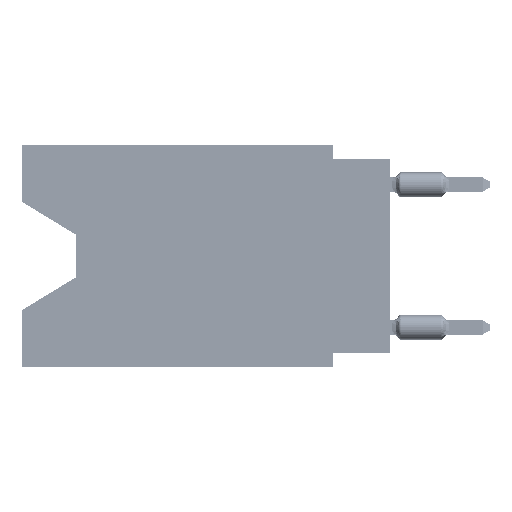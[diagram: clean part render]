
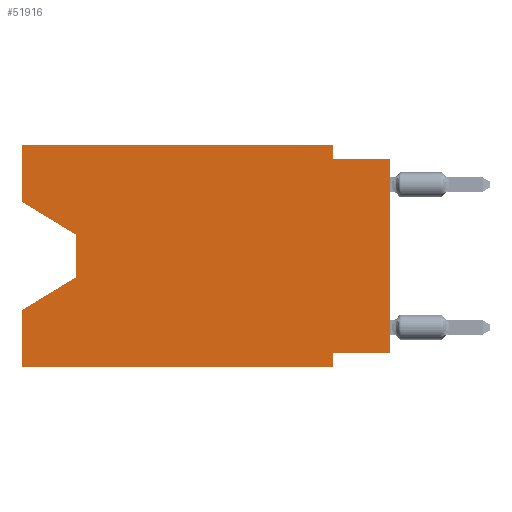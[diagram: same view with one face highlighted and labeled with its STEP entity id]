
A CAD part, left-side view. The second image highlights one B-rep face of the part: STEP entity #51916.
In plain terms, the highlighted planar face has unit normal (-1, 0, 0).
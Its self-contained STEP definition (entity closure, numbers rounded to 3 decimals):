
#1015 = CARTESIAN_POINT ( 'NONE',  ( 0., 13.97, -5.893 ) ) ;
#3054 = ORIENTED_EDGE ( 'NONE', *, *, #58920, .F. ) ;
#4257 = CARTESIAN_POINT ( 'NONE',  ( 0., 2.54, -9.906 ) ) ;
#5154 = DIRECTION ( 'NONE',  ( 0., 1., 0. ) ) ;
#5329 = LINE ( 'NONE', #80528, #53847 ) ;
#5830 = ORIENTED_EDGE ( 'NONE', *, *, #5962, .T. ) ;
#5930 = CARTESIAN_POINT ( 'NONE',  ( 0., 13.97, -4.013 ) ) ;
#5962 = EDGE_CURVE ( 'NONE', #19343, #60564, #78699, .T. ) ;
#6629 = DIRECTION ( 'NONE',  ( 0., 0., -1. ) ) ;
#7270 = LINE ( 'NONE', #87373, #84449 ) ;
#8302 = CARTESIAN_POINT ( 'NONE',  ( 0., 16.383, 0. ) ) ;
#9370 = DIRECTION ( 'NONE',  ( 1., 0., 0. ) ) ;
#10748 = CARTESIAN_POINT ( 'NONE',  ( 0., 13.97, -4.013 ) ) ;
#10751 = VERTEX_POINT ( 'NONE', #10748 ) ;
#11694 = EDGE_CURVE ( 'NONE', #61066, #87185, #7270, .T. ) ;
#11772 = VERTEX_POINT ( 'NONE', #76270 ) ;
#12384 = CARTESIAN_POINT ( 'NONE',  ( 0., 16.383, -7.36 ) ) ;
#12466 = VECTOR ( 'NONE', #78493, 1000. ) ;
#12744 = LINE ( 'NONE', #39727, #85848 ) ;
#13814 = ORIENTED_EDGE ( 'NONE', *, *, #39650, .F. ) ;
#13890 = ORIENTED_EDGE ( 'NONE', *, *, #84920, .F. ) ;
#14272 = LINE ( 'NONE', #1015, #20615 ) ;
#15813 = DIRECTION ( 'NONE',  ( 0., 0., 1. ) ) ;
#17654 = CARTESIAN_POINT ( 'NONE',  ( 0., 0., 0. ) ) ;
#18183 = CARTESIAN_POINT ( 'NONE',  ( 0., 2.54, -0.635 ) ) ;
#18396 = DIRECTION ( 'NONE',  ( 0., 0., -1. ) ) ;
#19343 = VERTEX_POINT ( 'NONE', #85067 ) ;
#19633 = VECTOR ( 'NONE', #85507, 1000. ) ;
#20615 = VECTOR ( 'NONE', #20919, 1000. ) ;
#20919 = DIRECTION ( 'NONE',  ( 0., 0.855, -0.519 ) ) ;
#21635 = EDGE_LOOP ( 'NONE', ( #86203, #53782, #53227, #3054, #43711, #22647, #13890, #5830, #42710, #52618, #77926, #13814 ) ) ;
#22647 = ORIENTED_EDGE ( 'NONE', *, *, #80457, .F. ) ;
#23345 = VECTOR ( 'NONE', #18396, 1000. ) ;
#24529 = LINE ( 'NONE', #46597, #12466 ) ;
#24726 = EDGE_CURVE ( 'NONE', #52031, #60564, #65137, .T. ) ;
#26306 = VECTOR ( 'NONE', #47828, 1000. ) ;
#27194 = DIRECTION ( 'NONE',  ( 0., -1., 0. ) ) ;
#29305 = EDGE_CURVE ( 'NONE', #10751, #38567, #58609, .T. ) ;
#29520 = LINE ( 'NONE', #8302, #60206 ) ;
#30520 = CARTESIAN_POINT ( 'NONE',  ( 0., 16.383, -9.906 ) ) ;
#30867 = EDGE_CURVE ( 'NONE', #43403, #10751, #24529, .T. ) ;
#31519 = CARTESIAN_POINT ( 'NONE',  ( 0., 0., -0.635 ) ) ;
#32839 = VERTEX_POINT ( 'NONE', #30520 ) ;
#36161 = VERTEX_POINT ( 'NONE', #47802 ) ;
#38349 = CARTESIAN_POINT ( 'NONE',  ( 0., 0., -9.271 ) ) ;
#38567 = VERTEX_POINT ( 'NONE', #83054 ) ;
#39650 = EDGE_CURVE ( 'NONE', #43403, #61066, #29520, .T. ) ;
#39727 = CARTESIAN_POINT ( 'NONE',  ( 0., 16.383, -9.906 ) ) ;
#42710 = ORIENTED_EDGE ( 'NONE', *, *, #24726, .F. ) ;
#42998 = FACE_OUTER_BOUND ( 'NONE', #21635, .T. ) ;
#43403 = VERTEX_POINT ( 'NONE', #57144 ) ;
#43711 = ORIENTED_EDGE ( 'NONE', *, *, #83452, .T. ) ;
#46597 = CARTESIAN_POINT ( 'NONE',  ( 0., 16.383, -2.546 ) ) ;
#47802 = CARTESIAN_POINT ( 'NONE',  ( 0., 2.54, -9.906 ) ) ;
#47828 = DIRECTION ( 'NONE',  ( 0., 0., 1. ) ) ;
#50363 = CARTESIAN_POINT ( 'NONE',  ( 0., 0., -0.635 ) ) ;
#50866 = EDGE_CURVE ( 'NONE', #87185, #52031, #5329, .T. ) ;
#51916 = ADVANCED_FACE ( 'NONE', ( #42998 ), #55400, .F. ) ;
#52031 = VERTEX_POINT ( 'NONE', #18183 ) ;
#52101 = VECTOR ( 'NONE', #5154, 1000. ) ;
#52387 = DIRECTION ( 'NONE',  ( 0., 0., -1. ) ) ;
#52618 = ORIENTED_EDGE ( 'NONE', *, *, #50866, .F. ) ;
#53227 = ORIENTED_EDGE ( 'NONE', *, *, #81063, .T. ) ;
#53782 = ORIENTED_EDGE ( 'NONE', *, *, #29305, .T. ) ;
#53847 = VECTOR ( 'NONE', #6629, 1000. ) ;
#54454 = LINE ( 'NONE', #81470, #26306 ) ;
#55400 = PLANE ( 'NONE',  #73818 ) ;
#56022 = CARTESIAN_POINT ( 'NONE',  ( 0., 16.383, 0. ) ) ;
#57144 = CARTESIAN_POINT ( 'NONE',  ( 0., 16.383, -2.546 ) ) ;
#58218 = CARTESIAN_POINT ( 'NONE',  ( 0., 2.54, 0. ) ) ;
#58609 = LINE ( 'NONE', #5930, #82955 ) ;
#58920 = EDGE_CURVE ( 'NONE', #32839, #68118, #54454, .T. ) ;
#60206 = VECTOR ( 'NONE', #15813, 1000. ) ;
#60564 = VERTEX_POINT ( 'NONE', #50363 ) ;
#61066 = VERTEX_POINT ( 'NONE', #56022 ) ;
#62784 = VECTOR ( 'NONE', #71624, 1000. ) ;
#65137 = LINE ( 'NONE', #31519, #19633 ) ;
#66722 = DIRECTION ( 'NONE',  ( 0., -1., 0. ) ) ;
#68118 = VERTEX_POINT ( 'NONE', #12384 ) ;
#71624 = DIRECTION ( 'NONE',  ( 0., 0., 1. ) ) ;
#73268 = LINE ( 'NONE', #38349, #52101 ) ;
#73818 = AXIS2_PLACEMENT_3D ( 'NONE', #77055, #9370, #75320 ) ;
#75320 = DIRECTION ( 'NONE',  ( 0., 0., -1. ) ) ;
#76270 = CARTESIAN_POINT ( 'NONE',  ( 0., 2.54, -9.271 ) ) ;
#77055 = CARTESIAN_POINT ( 'NONE',  ( 0., 16.383, 0. ) ) ;
#77926 = ORIENTED_EDGE ( 'NONE', *, *, #11694, .F. ) ;
#78493 = DIRECTION ( 'NONE',  ( 0., -0.855, -0.519 ) ) ;
#78699 = LINE ( 'NONE', #17654, #62784 ) ;
#80457 = EDGE_CURVE ( 'NONE', #11772, #36161, #86530, .T. ) ;
#80528 = CARTESIAN_POINT ( 'NONE',  ( 0., 2.54, 0. ) ) ;
#81063 = EDGE_CURVE ( 'NONE', #38567, #68118, #14272, .T. ) ;
#81470 = CARTESIAN_POINT ( 'NONE',  ( 0., 16.383, 0. ) ) ;
#82955 = VECTOR ( 'NONE', #52387, 1000. ) ;
#83054 = CARTESIAN_POINT ( 'NONE',  ( 0., 13.97, -5.893 ) ) ;
#83452 = EDGE_CURVE ( 'NONE', #32839, #36161, #12744, .T. ) ;
#84449 = VECTOR ( 'NONE', #27194, 1000. ) ;
#84920 = EDGE_CURVE ( 'NONE', #19343, #11772, #73268, .T. ) ;
#85067 = CARTESIAN_POINT ( 'NONE',  ( 0., 0., -9.271 ) ) ;
#85507 = DIRECTION ( 'NONE',  ( 0., -1., 0. ) ) ;
#85848 = VECTOR ( 'NONE', #66722, 1000. ) ;
#86203 = ORIENTED_EDGE ( 'NONE', *, *, #30867, .T. ) ;
#86530 = LINE ( 'NONE', #4257, #23345 ) ;
#87185 = VERTEX_POINT ( 'NONE', #58218 ) ;
#87373 = CARTESIAN_POINT ( 'NONE',  ( 0., 16.383, 0. ) ) ;
